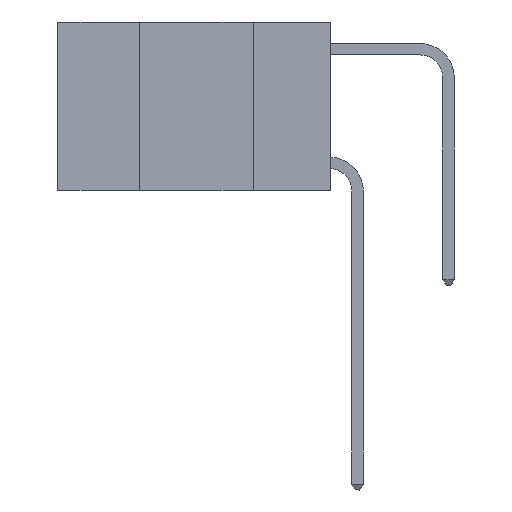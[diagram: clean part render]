
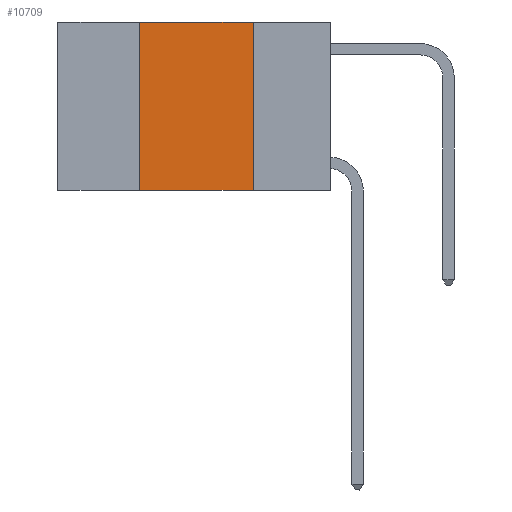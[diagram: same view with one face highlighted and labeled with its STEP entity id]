
A CAD part, left-side view. The second image highlights one B-rep face of the part: STEP entity #10709.
In plain terms, the highlighted planar face has unit normal (-1, 0, 0).
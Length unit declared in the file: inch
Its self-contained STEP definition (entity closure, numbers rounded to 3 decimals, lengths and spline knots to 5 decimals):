
#564 = EDGE_CURVE ( 'NONE', #1098, #6590, #4710, .T. ) ;
#1098 = VERTEX_POINT ( 'NONE', #1193 ) ;
#1161 = EDGE_CURVE ( 'NONE', #1098, #11274, #13849, .T. ) ;
#1193 = CARTESIAN_POINT ( 'NONE',  ( 0., 0.42, -0.37 ) ) ;
#1263 = VECTOR ( 'NONE', #8854, 39.37008 ) ;
#1361 = ORIENTED_EDGE ( 'NONE', *, *, #564, .F. ) ;
#1493 = EDGE_LOOP ( 'NONE', ( #11627, #11484, #1361, #5153 ) ) ;
#1884 = DIRECTION ( 'NONE',  ( 0., 0., -1. ) ) ;
#1978 = CARTESIAN_POINT ( 'NONE',  ( 0., 0.6, 0. ) ) ;
#2211 = VECTOR ( 'NONE', #5659, 39.37008 ) ;
#2551 = EDGE_CURVE ( 'NONE', #6590, #11322, #12929, .T. ) ;
#2921 = AXIS2_PLACEMENT_3D ( 'NONE', #12444, #6369, #1884 ) ;
#4616 = EDGE_CURVE ( 'NONE', #11322, #11274, #14771, .T. ) ;
#4710 = LINE ( 'NONE', #6965, #15066 ) ;
#5153 = ORIENTED_EDGE ( 'NONE', *, *, #1161, .T. ) ;
#5659 = DIRECTION ( 'NONE',  ( 0., -1., 0. ) ) ;
#5713 = CARTESIAN_POINT ( 'NONE',  ( 0., 0.42, 0. ) ) ;
#6369 = DIRECTION ( 'NONE',  ( 1., 0., 0. ) ) ;
#6590 = VERTEX_POINT ( 'NONE', #5713 ) ;
#6965 = CARTESIAN_POINT ( 'NONE',  ( 0., 0.42, 0. ) ) ;
#7572 = PLANE ( 'NONE',  #2921 ) ;
#8362 = CARTESIAN_POINT ( 'NONE',  ( 0., 0.17, -0.37 ) ) ;
#8854 = DIRECTION ( 'NONE',  ( 0., 0., -1. ) ) ;
#9731 = CARTESIAN_POINT ( 'NONE',  ( 0., 0.17, 0. ) ) ;
#10709 = ADVANCED_FACE ( 'NONE', ( #11018 ), #7572, .F. ) ;
#11018 = FACE_OUTER_BOUND ( 'NONE', #1493, .T. ) ;
#11274 = VERTEX_POINT ( 'NONE', #8362 ) ;
#11322 = VERTEX_POINT ( 'NONE', #9731 ) ;
#11484 = ORIENTED_EDGE ( 'NONE', *, *, #2551, .F. ) ;
#11627 = ORIENTED_EDGE ( 'NONE', *, *, #4616, .F. ) ;
#12444 = CARTESIAN_POINT ( 'NONE',  ( 0., 0.6, 0. ) ) ;
#12929 = LINE ( 'NONE', #1978, #2211 ) ;
#13783 = CARTESIAN_POINT ( 'NONE',  ( 0., 0.6, -0.37 ) ) ;
#13849 = LINE ( 'NONE', #13783, #13964 ) ;
#13964 = VECTOR ( 'NONE', #14604, 39.37008 ) ;
#14604 = DIRECTION ( 'NONE',  ( 0., -1., 0. ) ) ;
#14771 = LINE ( 'NONE', #15001, #1263 ) ;
#15001 = CARTESIAN_POINT ( 'NONE',  ( 0., 0.17, 0. ) ) ;
#15066 = VECTOR ( 'NONE', #15748, 39.37008 ) ;
#15748 = DIRECTION ( 'NONE',  ( 0., 0., 1. ) ) ;
